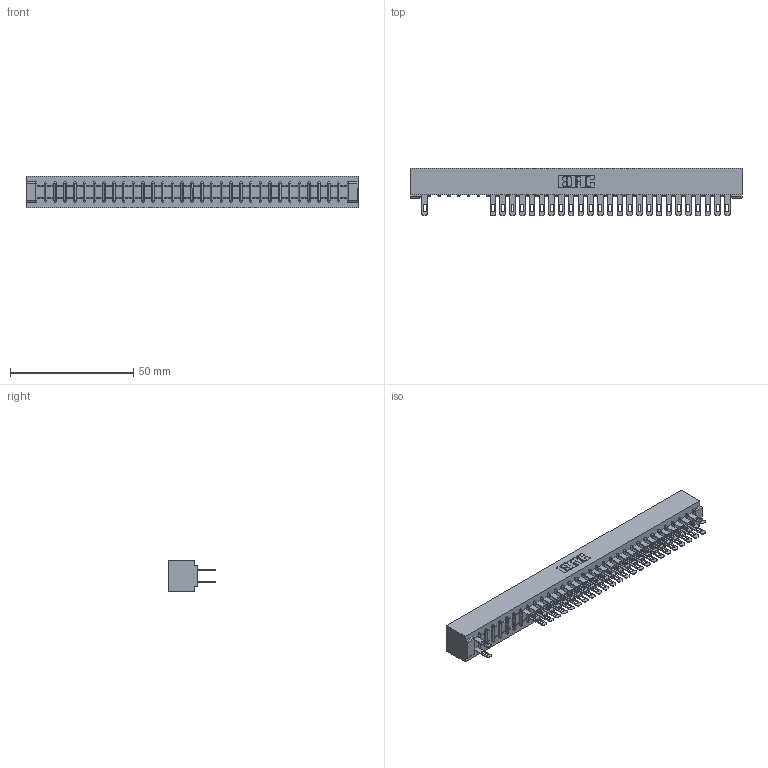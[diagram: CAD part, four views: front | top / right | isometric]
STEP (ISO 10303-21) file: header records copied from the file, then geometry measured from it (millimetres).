
FILE_DESCRIPTION (( 'STEP AP203' ), '1' );
FILE_NAME ('307-064-500-201.STEP', '2018-08-06T09:49:16', ( '' ), ( '' ), 'SwSTEP 2.0', 'SolidWorks 2016', '' );
FILE_SCHEMA (( 'CONFIG_CONTROL_DESIGN' ));
Length unit declared in the file: inch
Products named in the file (3): 307-064-500-201; 307 Part_No Mounting Lugs; 307-290-001_500
Assembly tree (52 placements, depth 2):
  307-064-500-201
    307 Part_No Mounting Lugs
    307-290-001_500  x51
Bounding box: 134.67 x 19.18 x 12.7 mm (x, y, z)
Volume: 14775.1 mm3; surface area: 17897.7 mm2
Topology: 52 solids, 52 shells, 2619 faces, 7345 edges, 4738 vertices
Faces by surface type: plane 1674, cylinder 879, sphere 66
Entity records: 28970 total; most frequent: CARTESIAN_POINT 4791, ORIENTED_EDGE 4758, DIRECTION 4685, EDGE_CURVE 2379, LINE 1821, VECTOR 1821, VERTEX_POINT 1538, AXIS2_PLACEMENT_3D 1432
